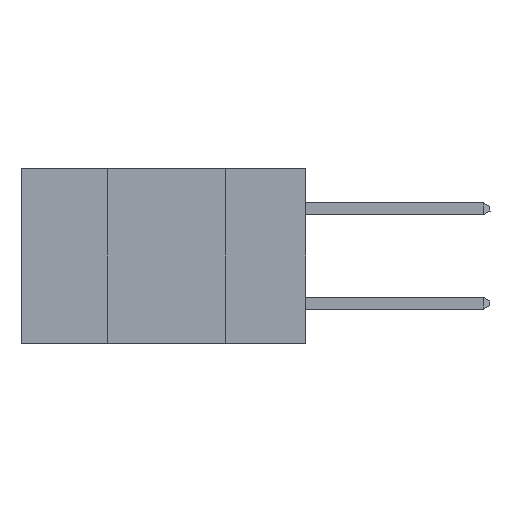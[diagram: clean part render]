
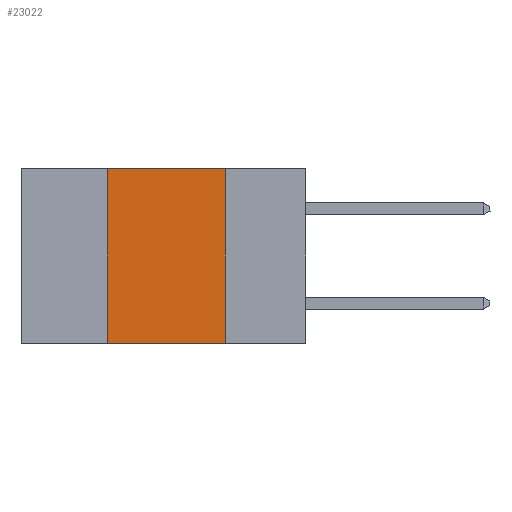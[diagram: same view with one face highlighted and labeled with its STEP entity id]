
A CAD part, left-side view. The second image highlights one B-rep face of the part: STEP entity #23022.
In plain terms, the highlighted planar face has unit normal (-1, 0, 0).
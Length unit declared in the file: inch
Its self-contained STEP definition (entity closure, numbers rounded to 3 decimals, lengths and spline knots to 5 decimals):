
#921 = LINE ( 'NONE', #18157, #7170 ) ;
#1189 = ORIENTED_EDGE ( 'NONE', *, *, #24606, .F. ) ;
#1590 = CARTESIAN_POINT ( 'NONE',  ( 0., 0.6, 0. ) ) ;
#1750 = DIRECTION ( 'NONE',  ( 0., -1., 0. ) ) ;
#1874 = VECTOR ( 'NONE', #17009, 39.37008 ) ;
#2791 = AXIS2_PLACEMENT_3D ( 'NONE', #1590, #15996, #3716 ) ;
#3716 = DIRECTION ( 'NONE',  ( 0., 0., -1. ) ) ;
#4456 = ORIENTED_EDGE ( 'NONE', *, *, #7203, .F. ) ;
#4753 = DIRECTION ( 'NONE',  ( 0., 0., -1. ) ) ;
#5519 = ORIENTED_EDGE ( 'NONE', *, *, #22677, .F. ) ;
#5701 = LINE ( 'NONE', #20708, #21106 ) ;
#5749 = PLANE ( 'NONE',  #2791 ) ;
#7170 = VECTOR ( 'NONE', #1750, 39.37008 ) ;
#7203 = EDGE_CURVE ( 'NONE', #15116, #13821, #921, .T. ) ;
#7791 = EDGE_CURVE ( 'NONE', #13160, #10141, #18222, .T. ) ;
#9356 = ORIENTED_EDGE ( 'NONE', *, *, #7791, .T. ) ;
#10141 = VERTEX_POINT ( 'NONE', #23960 ) ;
#11302 = EDGE_LOOP ( 'NONE', ( #1189, #4456, #5519, #9356 ) ) ;
#12502 = CARTESIAN_POINT ( 'NONE',  ( 0., 0.42, 0. ) ) ;
#13160 = VERTEX_POINT ( 'NONE', #21210 ) ;
#13821 = VERTEX_POINT ( 'NONE', #24654 ) ;
#14978 = CARTESIAN_POINT ( 'NONE',  ( 0., 0.6, -0.37 ) ) ;
#15116 = VERTEX_POINT ( 'NONE', #12502 ) ;
#15996 = DIRECTION ( 'NONE',  ( 1., 0., 0. ) ) ;
#16460 = VECTOR ( 'NONE', #4753, 39.37008 ) ;
#17009 = DIRECTION ( 'NONE',  ( 0., -1., 0. ) ) ;
#18157 = CARTESIAN_POINT ( 'NONE',  ( 0., 0.6, 0. ) ) ;
#18222 = LINE ( 'NONE', #14978, #1874 ) ;
#18373 = FACE_OUTER_BOUND ( 'NONE', #11302, .T. ) ;
#18949 = CARTESIAN_POINT ( 'NONE',  ( 0., 0.17, 0. ) ) ;
#20708 = CARTESIAN_POINT ( 'NONE',  ( 0., 0.42, 0. ) ) ;
#21106 = VECTOR ( 'NONE', #22651, 39.37008 ) ;
#21210 = CARTESIAN_POINT ( 'NONE',  ( 0., 0.42, -0.37 ) ) ;
#21638 = LINE ( 'NONE', #18949, #16460 ) ;
#22651 = DIRECTION ( 'NONE',  ( 0., 0., 1. ) ) ;
#22677 = EDGE_CURVE ( 'NONE', #13160, #15116, #5701, .T. ) ;
#23022 = ADVANCED_FACE ( 'NONE', ( #18373 ), #5749, .F. ) ;
#23960 = CARTESIAN_POINT ( 'NONE',  ( 0., 0.17, -0.37 ) ) ;
#24606 = EDGE_CURVE ( 'NONE', #13821, #10141, #21638, .T. ) ;
#24654 = CARTESIAN_POINT ( 'NONE',  ( 0., 0.17, 0. ) ) ;
